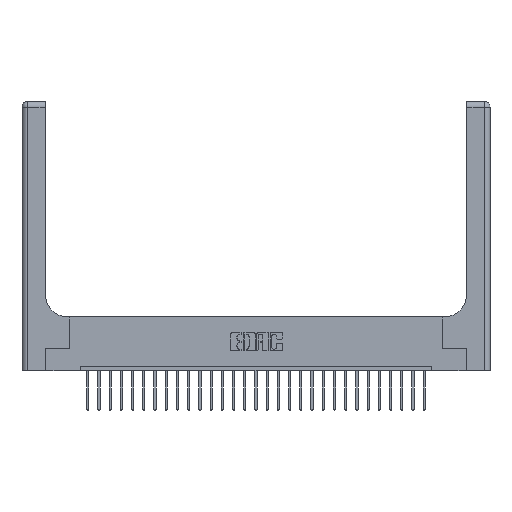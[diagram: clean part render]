
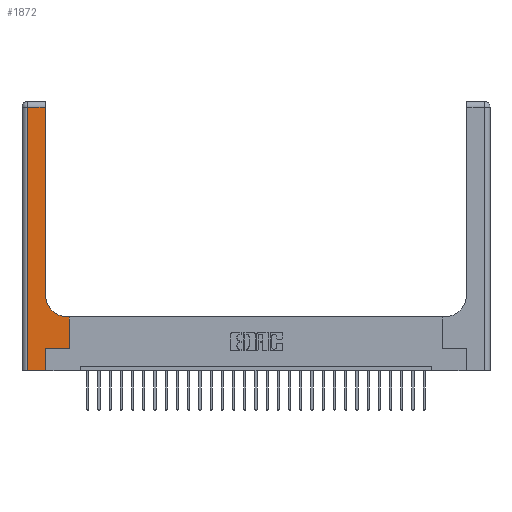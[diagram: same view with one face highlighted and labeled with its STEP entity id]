
A CAD part, top view. The second image highlights one B-rep face of the part: STEP entity #1872.
In plain terms, the highlighted planar face has unit normal (0, 0, 1).
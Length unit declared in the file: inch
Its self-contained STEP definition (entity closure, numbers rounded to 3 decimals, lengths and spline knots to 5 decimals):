
#312 = CARTESIAN_POINT ( 'NONE',  ( 0.26, 0.6, 0.37 ) ) ;
#1132 = AXIS2_PLACEMENT_3D ( 'NONE', #22231, #2578, #18389 ) ;
#1872 = ADVANCED_FACE ( 'NONE', ( #3605 ), #6091, .F. ) ;
#2024 = LINE ( 'NONE', #312, #18623 ) ;
#2302 = DIRECTION ( 'NONE',  ( 1., 0., 0. ) ) ;
#2578 = DIRECTION ( 'NONE',  ( 0., 0., -1. ) ) ;
#3454 = CARTESIAN_POINT ( 'NONE',  ( 0.06, 3., 0.37 ) ) ;
#3605 = FACE_OUTER_BOUND ( 'NONE', #25538, .T. ) ;
#3936 = DIRECTION ( 'NONE',  ( 0., 0., -1. ) ) ;
#4235 = CARTESIAN_POINT ( 'NONE',  ( 0.528, 0.6, 0.37 ) ) ;
#4263 = LINE ( 'NONE', #24594, #19571 ) ;
#4375 = ORIENTED_EDGE ( 'NONE', *, *, #6057, .T. ) ;
#5358 = DIRECTION ( 'NONE',  ( 1., 0., 0. ) ) ;
#5625 = VERTEX_POINT ( 'NONE', #12394 ) ;
#5661 = ORIENTED_EDGE ( 'NONE', *, *, #21766, .T. ) ;
#5829 = CARTESIAN_POINT ( 'NONE',  ( 0.06, 0., 0.37 ) ) ;
#6057 = EDGE_CURVE ( 'NONE', #5625, #21922, #4263, .T. ) ;
#6091 = PLANE ( 'NONE',  #13228 ) ;
#6501 = LINE ( 'NONE', #14155, #21213 ) ;
#6652 = EDGE_CURVE ( 'NONE', #21922, #8308, #12338, .T. ) ;
#6908 = EDGE_CURVE ( 'NONE', #12416, #19080, #11671, .T. ) ;
#7736 = CARTESIAN_POINT ( 'NONE',  ( 0.265, 0.25, 0.37 ) ) ;
#7985 = ORIENTED_EDGE ( 'NONE', *, *, #20568, .T. ) ;
#8089 = DIRECTION ( 'NONE',  ( -1., 0., 0. ) ) ;
#8308 = VERTEX_POINT ( 'NONE', #20546 ) ;
#8569 = DIRECTION ( 'NONE',  ( 0., 1., 0. ) ) ;
#8701 = CIRCLE ( 'NONE', #1132, 0.25 ) ;
#9922 = CARTESIAN_POINT ( 'NONE',  ( 0., 3., 0.37 ) ) ;
#9988 = VECTOR ( 'NONE', #5358, 39.37008 ) ;
#11671 = LINE ( 'NONE', #22225, #20446 ) ;
#12180 = LINE ( 'NONE', #3454, #25942 ) ;
#12338 = LINE ( 'NONE', #23167, #20470 ) ;
#12394 = CARTESIAN_POINT ( 'NONE',  ( 0.26, 0.85, 0.37 ) ) ;
#12416 = VERTEX_POINT ( 'NONE', #7736 ) ;
#12545 = EDGE_CURVE ( 'NONE', #20870, #12416, #12660, .T. ) ;
#12572 = EDGE_CURVE ( 'NONE', #21608, #24194, #2024, .T. ) ;
#12660 = LINE ( 'NONE', #14243, #22042 ) ;
#12701 = CARTESIAN_POINT ( 'NONE',  ( 0.51, 0.6, 0.37 ) ) ;
#13228 = AXIS2_PLACEMENT_3D ( 'NONE', #9922, #3936, #8089 ) ;
#13561 = CARTESIAN_POINT ( 'NONE',  ( 0., 0., 0.37 ) ) ;
#13563 = DIRECTION ( 'NONE',  ( 0., -1., 0. ) ) ;
#13764 = LINE ( 'NONE', #13561, #9988 ) ;
#14155 = CARTESIAN_POINT ( 'NONE',  ( 0.528, 0.25, 0.37 ) ) ;
#14243 = CARTESIAN_POINT ( 'NONE',  ( 0.265, 0., 0.37 ) ) ;
#14339 = DIRECTION ( 'NONE',  ( -1., 0., 0. ) ) ;
#15052 = ORIENTED_EDGE ( 'NONE', *, *, #12545, .T. ) ;
#16206 = DIRECTION ( 'NONE',  ( 0., 1., 0. ) ) ;
#16907 = ORIENTED_EDGE ( 'NONE', *, *, #6652, .T. ) ;
#17607 = DIRECTION ( 'NONE',  ( -1., 0., 0. ) ) ;
#18006 = ORIENTED_EDGE ( 'NONE', *, *, #6908, .T. ) ;
#18088 = ORIENTED_EDGE ( 'NONE', *, *, #24513, .T. ) ;
#18327 = VERTEX_POINT ( 'NONE', #5829 ) ;
#18389 = DIRECTION ( 'NONE',  ( 1., 0., 0. ) ) ;
#18623 = VECTOR ( 'NONE', #14339, 39.37008 ) ;
#19080 = VERTEX_POINT ( 'NONE', #24345 ) ;
#19571 = VECTOR ( 'NONE', #8569, 39.37008 ) ;
#19984 = DIRECTION ( 'NONE',  ( 0., 1., 0. ) ) ;
#20141 = ORIENTED_EDGE ( 'NONE', *, *, #12572, .T. ) ;
#20446 = VECTOR ( 'NONE', #2302, 39.37008 ) ;
#20470 = VECTOR ( 'NONE', #17607, 39.37008 ) ;
#20546 = CARTESIAN_POINT ( 'NONE',  ( 0.06, 2.94, 0.37 ) ) ;
#20568 = EDGE_CURVE ( 'NONE', #18327, #20870, #13764, .T. ) ;
#20608 = ORIENTED_EDGE ( 'NONE', *, *, #25132, .T. ) ;
#20870 = VERTEX_POINT ( 'NONE', #25497 ) ;
#21213 = VECTOR ( 'NONE', #16206, 39.37008 ) ;
#21608 = VERTEX_POINT ( 'NONE', #4235 ) ;
#21766 = EDGE_CURVE ( 'NONE', #24194, #5625, #8701, .T. ) ;
#21922 = VERTEX_POINT ( 'NONE', #24945 ) ;
#22042 = VECTOR ( 'NONE', #19984, 39.37008 ) ;
#22225 = CARTESIAN_POINT ( 'NONE',  ( 0.265, 0.25, 0.37 ) ) ;
#22231 = CARTESIAN_POINT ( 'NONE',  ( 0.51, 0.85, 0.37 ) ) ;
#23167 = CARTESIAN_POINT ( 'NONE',  ( 0., 2.94, 0.37 ) ) ;
#24194 = VERTEX_POINT ( 'NONE', #12701 ) ;
#24345 = CARTESIAN_POINT ( 'NONE',  ( 0.528, 0.25, 0.37 ) ) ;
#24513 = EDGE_CURVE ( 'NONE', #8308, #18327, #12180, .T. ) ;
#24594 = CARTESIAN_POINT ( 'NONE',  ( 0.26, 3., 0.37 ) ) ;
#24945 = CARTESIAN_POINT ( 'NONE',  ( 0.26, 2.94, 0.37 ) ) ;
#25132 = EDGE_CURVE ( 'NONE', #19080, #21608, #6501, .T. ) ;
#25497 = CARTESIAN_POINT ( 'NONE',  ( 0.265, 0., 0.37 ) ) ;
#25538 = EDGE_LOOP ( 'NONE', ( #4375, #16907, #18088, #7985, #15052, #18006, #20608, #20141, #5661 ) ) ;
#25942 = VECTOR ( 'NONE', #13563, 39.37008 ) ;
